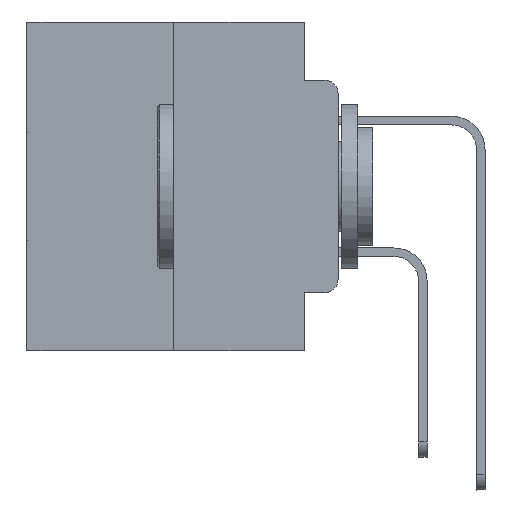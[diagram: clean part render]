
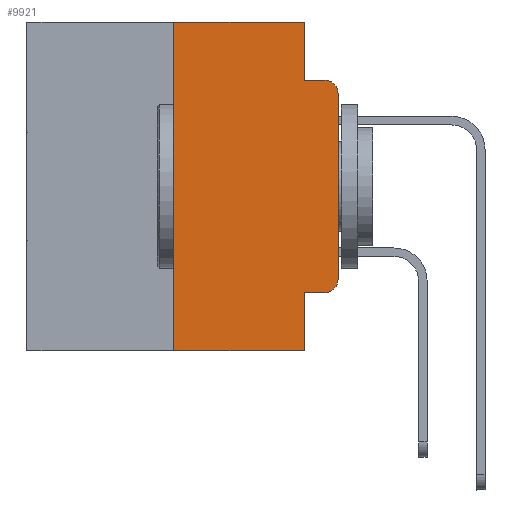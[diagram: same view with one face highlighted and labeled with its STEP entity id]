
A CAD part, left-side view. The second image highlights one B-rep face of the part: STEP entity #9921.
In plain terms, the highlighted planar face has unit normal (-1, 0, 0).
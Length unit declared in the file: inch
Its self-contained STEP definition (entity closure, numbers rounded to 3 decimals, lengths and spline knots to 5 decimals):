
#32 = CARTESIAN_POINT ( 'NONE',  ( 0., 0.473, 0. ) ) ;
#268 = EDGE_CURVE ( 'NONE', #20098, #21382, #638, .T. ) ;
#638 = LINE ( 'NONE', #29739, #6607 ) ;
#905 = CARTESIAN_POINT ( 'NONE',  ( 0., 0.02, -0.0885 ) ) ;
#1996 = EDGE_CURVE ( 'NONE', #21382, #21280, #8733, .T. ) ;
#2159 = LINE ( 'NONE', #15777, #20728 ) ;
#2176 = VECTOR ( 'NONE', #17468, 39.37008 ) ;
#2301 = ORIENTED_EDGE ( 'NONE', *, *, #12875, .F. ) ;
#2454 = PLANE ( 'NONE',  #7476 ) ;
#2477 = DIRECTION ( 'NONE',  ( 0., 0., -1. ) ) ;
#2677 = VERTEX_POINT ( 'NONE', #2947 ) ;
#2947 = CARTESIAN_POINT ( 'NONE',  ( 0., 0.051, -0.5 ) ) ;
#3234 = CARTESIAN_POINT ( 'NONE',  ( 0., 0.02, -0.1085 ) ) ;
#3922 = ORIENTED_EDGE ( 'NONE', *, *, #26705, .F. ) ;
#5030 = CARTESIAN_POINT ( 'NONE',  ( 0., 0.473, 0. ) ) ;
#5096 = CARTESIAN_POINT ( 'NONE',  ( 0., 0.051, 0. ) ) ;
#5403 = EDGE_LOOP ( 'NONE', ( #24852, #30979, #6643, #27023, #2301, #22298, #28484, #3922, #23793, #29912 ) ) ;
#5424 = EDGE_CURVE ( 'NONE', #30369, #21280, #17200, .T. ) ;
#5789 = DIRECTION ( 'NONE',  ( 0., 0., -1. ) ) ;
#6601 = VERTEX_POINT ( 'NONE', #23470 ) ;
#6607 = VECTOR ( 'NONE', #2477, 39.37008 ) ;
#6643 = ORIENTED_EDGE ( 'NONE', *, *, #1996, .F. ) ;
#6723 = VECTOR ( 'NONE', #9902, 39.37008 ) ;
#7070 = EDGE_CURVE ( 'NONE', #26254, #30369, #18944, .T. ) ;
#7152 = VERTEX_POINT ( 'NONE', #16304 ) ;
#7476 = AXIS2_PLACEMENT_3D ( 'NONE', #5030, #24130, #9950 ) ;
#7479 = DIRECTION ( 'NONE',  ( 0., 0., 1. ) ) ;
#8028 = VERTEX_POINT ( 'NONE', #9720 ) ;
#8031 = AXIS2_PLACEMENT_3D ( 'NONE', #28367, #14386, #30673 ) ;
#8400 = VECTOR ( 'NONE', #15696, 39.37008 ) ;
#8733 = LINE ( 'NONE', #15359, #8400 ) ;
#9720 = CARTESIAN_POINT ( 'NONE',  ( 0., 0.02, -0.4115 ) ) ;
#9902 = DIRECTION ( 'NONE',  ( 0., 0., -1. ) ) ;
#9921 = ADVANCED_FACE ( 'NONE', ( #27051 ), #2454, .F. ) ;
#9950 = DIRECTION ( 'NONE',  ( 0., 0., -1. ) ) ;
#12043 = CARTESIAN_POINT ( 'NONE',  ( 0., 0.051, -0.4115 ) ) ;
#12368 = DIRECTION ( 'NONE',  ( 0., -1., 0. ) ) ;
#12875 = EDGE_CURVE ( 'NONE', #6601, #20098, #15994, .T. ) ;
#13030 = CARTESIAN_POINT ( 'NONE',  ( 0., 0., -0.3915 ) ) ;
#14386 = DIRECTION ( 'NONE',  ( -1., 0., 0. ) ) ;
#14694 = LINE ( 'NONE', #5096, #6723 ) ;
#15061 = CARTESIAN_POINT ( 'NONE',  ( 0., 0.051, 0. ) ) ;
#15359 = CARTESIAN_POINT ( 'NONE',  ( 0., 0.051, -0.0885 ) ) ;
#15696 = DIRECTION ( 'NONE',  ( 0., -1., 0. ) ) ;
#15777 = CARTESIAN_POINT ( 'NONE',  ( 0., 0.051, -0.4115 ) ) ;
#15976 = VECTOR ( 'NONE', #12368, 39.37008 ) ;
#15994 = LINE ( 'NONE', #32, #2176 ) ;
#16172 = CARTESIAN_POINT ( 'NONE',  ( 0., 0.051, -0.0885 ) ) ;
#16179 = EDGE_CURVE ( 'NONE', #7152, #2677, #28351, .T. ) ;
#16304 = CARTESIAN_POINT ( 'NONE',  ( 0., 0.25, -0.5 ) ) ;
#17085 = AXIS2_PLACEMENT_3D ( 'NONE', #3234, #20155, #5789 ) ;
#17200 = CIRCLE ( 'NONE', #17085, 0.02 ) ;
#17468 = DIRECTION ( 'NONE',  ( 0., -1., 0. ) ) ;
#18154 = DIRECTION ( 'NONE',  ( 0., -1., 0. ) ) ;
#18250 = VECTOR ( 'NONE', #7479, 39.37008 ) ;
#18272 = CARTESIAN_POINT ( 'NONE',  ( 0., 0., 0. ) ) ;
#18944 = LINE ( 'NONE', #18272, #25109 ) ;
#19434 = CARTESIAN_POINT ( 'NONE',  ( 0., 0.25, 0. ) ) ;
#19610 = CARTESIAN_POINT ( 'NONE',  ( 0., 0., -0.1085 ) ) ;
#20098 = VERTEX_POINT ( 'NONE', #15061 ) ;
#20155 = DIRECTION ( 'NONE',  ( -1., 0., 0. ) ) ;
#20728 = VECTOR ( 'NONE', #18154, 39.37008 ) ;
#21280 = VERTEX_POINT ( 'NONE', #905 ) ;
#21382 = VERTEX_POINT ( 'NONE', #16172 ) ;
#22298 = ORIENTED_EDGE ( 'NONE', *, *, #29784, .F. ) ;
#23470 = CARTESIAN_POINT ( 'NONE',  ( 0., 0.25, 0. ) ) ;
#23597 = EDGE_CURVE ( 'NONE', #8028, #26254, #28087, .T. ) ;
#23793 = ORIENTED_EDGE ( 'NONE', *, *, #25150, .T. ) ;
#24130 = DIRECTION ( 'NONE',  ( 1., 0., 0. ) ) ;
#24852 = ORIENTED_EDGE ( 'NONE', *, *, #7070, .T. ) ;
#25109 = VECTOR ( 'NONE', #29700, 39.37008 ) ;
#25148 = LINE ( 'NONE', #19434, #18250 ) ;
#25150 = EDGE_CURVE ( 'NONE', #27247, #8028, #2159, .T. ) ;
#26254 = VERTEX_POINT ( 'NONE', #13030 ) ;
#26381 = CARTESIAN_POINT ( 'NONE',  ( 0., 0.473, -0.5 ) ) ;
#26705 = EDGE_CURVE ( 'NONE', #27247, #2677, #14694, .T. ) ;
#27023 = ORIENTED_EDGE ( 'NONE', *, *, #268, .F. ) ;
#27051 = FACE_OUTER_BOUND ( 'NONE', #5403, .T. ) ;
#27247 = VERTEX_POINT ( 'NONE', #12043 ) ;
#28087 = CIRCLE ( 'NONE', #8031, 0.02 ) ;
#28351 = LINE ( 'NONE', #26381, #15976 ) ;
#28367 = CARTESIAN_POINT ( 'NONE',  ( 0., 0.02, -0.3915 ) ) ;
#28484 = ORIENTED_EDGE ( 'NONE', *, *, #16179, .T. ) ;
#29700 = DIRECTION ( 'NONE',  ( 0., 0., 1. ) ) ;
#29739 = CARTESIAN_POINT ( 'NONE',  ( 0., 0.051, 0. ) ) ;
#29784 = EDGE_CURVE ( 'NONE', #7152, #6601, #25148, .T. ) ;
#29912 = ORIENTED_EDGE ( 'NONE', *, *, #23597, .T. ) ;
#30369 = VERTEX_POINT ( 'NONE', #19610 ) ;
#30673 = DIRECTION ( 'NONE',  ( 0., 0., -1. ) ) ;
#30979 = ORIENTED_EDGE ( 'NONE', *, *, #5424, .T. ) ;
